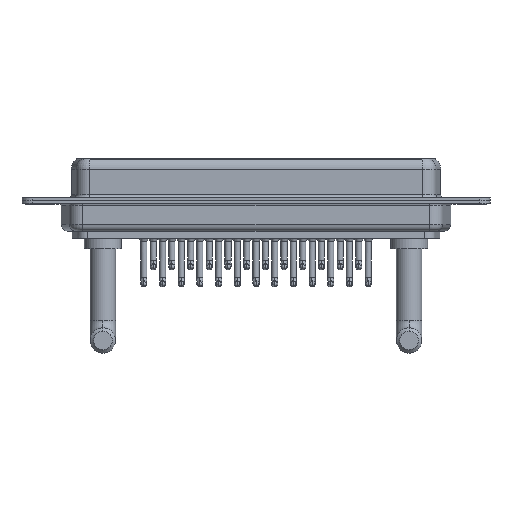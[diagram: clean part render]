
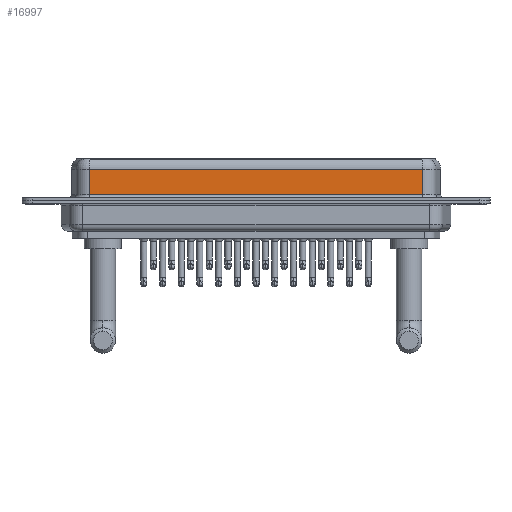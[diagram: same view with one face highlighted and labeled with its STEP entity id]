
A CAD part, front view. The second image highlights one B-rep face of the part: STEP entity #16997.
In plain terms, the highlighted planar face has unit normal (0, -1, 0).
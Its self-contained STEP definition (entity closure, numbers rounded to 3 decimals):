
#8 = LINE ( 'NONE', #3844, #19836 ) ;
#756 = LINE ( 'NONE', #16925, #22824 ) ;
#871 = DIRECTION ( 'NONE',  ( 1., 0., 0. ) ) ;
#928 = VERTEX_POINT ( 'NONE', #12647 ) ;
#1066 = VERTEX_POINT ( 'NONE', #21600 ) ;
#1425 = VECTOR ( 'NONE', #19737, 1000. ) ;
#1611 = EDGE_CURVE ( 'NONE', #928, #6945, #8, .T. ) ;
#1714 = DIRECTION ( 'NONE',  ( 0., 1., 0. ) ) ;
#1822 = CARTESIAN_POINT ( 'NONE',  ( 7.038, -3.95, 6.4 ) ) ;
#3064 = ORIENTED_EDGE ( 'NONE', *, *, #1611, .T. ) ;
#3192 = CARTESIAN_POINT ( 'NONE',  ( 56.462, -3.95, 0.9 ) ) ;
#3793 = FACE_OUTER_BOUND ( 'NONE', #7175, .T. ) ;
#3844 = CARTESIAN_POINT ( 'NONE',  ( 56.462, -3.95, 4.65 ) ) ;
#3845 = EDGE_CURVE ( 'NONE', #6945, #1066, #14487, .T. ) ;
#5897 = DIRECTION ( 'NONE',  ( 0., 0., -1. ) ) ;
#6945 = VERTEX_POINT ( 'NONE', #12114 ) ;
#7175 = EDGE_LOOP ( 'NONE', ( #16443, #3064, #13726, #16735 ) ) ;
#8723 = AXIS2_PLACEMENT_3D ( 'NONE', #17642, #1714, #20177 ) ;
#9114 = EDGE_CURVE ( 'NONE', #928, #14155, #12895, .T. ) ;
#10888 = PLANE ( 'NONE',  #8723 ) ;
#12114 = CARTESIAN_POINT ( 'NONE',  ( 7.038, -3.95, 4.65 ) ) ;
#12275 = VECTOR ( 'NONE', #5897, 1000. ) ;
#12647 = CARTESIAN_POINT ( 'NONE',  ( 56.462, -3.95, 4.65 ) ) ;
#12895 = LINE ( 'NONE', #21984, #12275 ) ;
#13726 = ORIENTED_EDGE ( 'NONE', *, *, #3845, .T. ) ;
#14033 = EDGE_CURVE ( 'NONE', #1066, #14155, #756, .T. ) ;
#14155 = VERTEX_POINT ( 'NONE', #3192 ) ;
#14487 = LINE ( 'NONE', #1822, #1425 ) ;
#16394 = DIRECTION ( 'NONE',  ( -1., 0., 0. ) ) ;
#16443 = ORIENTED_EDGE ( 'NONE', *, *, #9114, .F. ) ;
#16735 = ORIENTED_EDGE ( 'NONE', *, *, #14033, .T. ) ;
#16925 = CARTESIAN_POINT ( 'NONE',  ( 56.462, -3.95, 0.9 ) ) ;
#16997 = ADVANCED_FACE ( 'NONE', ( #3793 ), #10888, .F. ) ;
#17642 = CARTESIAN_POINT ( 'NONE',  ( 56.462, -3.95, 6.4 ) ) ;
#19737 = DIRECTION ( 'NONE',  ( 0., 0., -1. ) ) ;
#19836 = VECTOR ( 'NONE', #16394, 1000. ) ;
#20177 = DIRECTION ( 'NONE',  ( 0., 0., 1. ) ) ;
#21600 = CARTESIAN_POINT ( 'NONE',  ( 7.038, -3.95, 0.9 ) ) ;
#21984 = CARTESIAN_POINT ( 'NONE',  ( 56.462, -3.95, 6.4 ) ) ;
#22824 = VECTOR ( 'NONE', #871, 1000. ) ;
